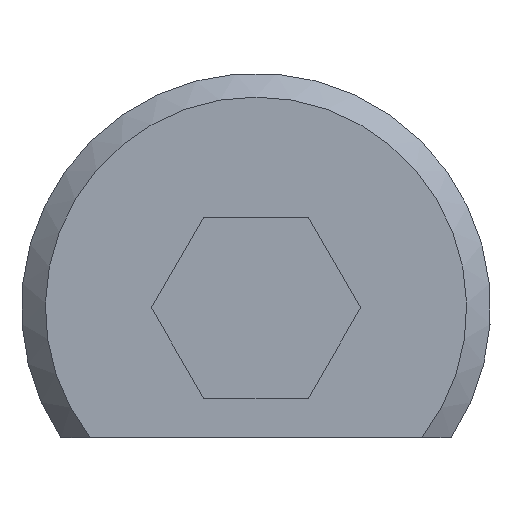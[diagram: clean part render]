
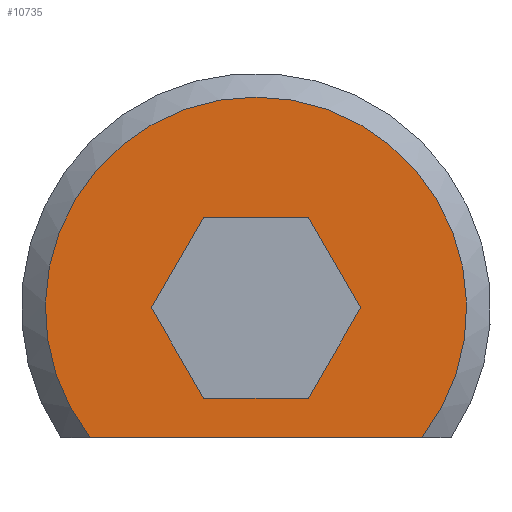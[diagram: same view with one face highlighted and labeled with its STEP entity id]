
A CAD part, left-side view. The second image highlights one B-rep face of the part: STEP entity #10735.
In plain terms, the highlighted planar face has unit normal (-1, 0, 0).
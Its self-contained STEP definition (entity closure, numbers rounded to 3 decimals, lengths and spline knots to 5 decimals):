
#2374 = CARTESIAN_POINT ( 'NONE',  ( -0.25, -0.26053, -0.20458 ) ) ;
#7805 = CARTESIAN_POINT ( 'NONE',  ( -0.25, -0.08223, 0.14242 ) ) ;
#7925 = CARTESIAN_POINT ( 'NONE',  ( -0.25, -0.16445, 0. ) ) ;
#10735 = ADVANCED_FACE ( 'NONE', ( #48228, #26675 ), #14291, .T. ) ;
#12114 = VERTEX_POINT ( 'NONE', #19685 ) ;
#14291 = PLANE ( 'NONE',  #78402 ) ;
#15123 = CARTESIAN_POINT ( 'NONE',  ( -0.25, 0.08223, 0.14242 ) ) ;
#15304 = DIRECTION ( 'NONE',  ( -1., 0., 0. ) ) ;
#15470 = VERTEX_POINT ( 'NONE', #93569 ) ;
#15492 = DIRECTION ( 'NONE',  ( 0., -1., 0. ) ) ;
#16878 = DIRECTION ( 'NONE',  ( 0., 0.5, -0.866 ) ) ;
#19685 = CARTESIAN_POINT ( 'NONE',  ( -0.25, -0.16445, 0. ) ) ;
#19991 = EDGE_CURVE ( 'NONE', #75004, #82267, #100222, .T. ) ;
#22116 = DIRECTION ( 'NONE',  ( 0., 0., 1. ) ) ;
#23734 = LINE ( 'NONE', #38439, #74412 ) ;
#24244 = ORIENTED_EDGE ( 'NONE', *, *, #19991, .F. ) ;
#25272 = CARTESIAN_POINT ( 'NONE',  ( -0.25, -0.08223, -0.14242 ) ) ;
#26675 = FACE_BOUND ( 'NONE', #87872, .T. ) ;
#28014 = EDGE_CURVE ( 'NONE', #12114, #42615, #59497, .T. ) ;
#29639 = ORIENTED_EDGE ( 'NONE', *, *, #64154, .T. ) ;
#32819 = EDGE_CURVE ( 'NONE', #15470, #101002, #70896, .T. ) ;
#33434 = EDGE_CURVE ( 'NONE', #91427, #12114, #78535, .T. ) ;
#33846 = DIRECTION ( 'NONE',  ( -1., 0., 0. ) ) ;
#35648 = CARTESIAN_POINT ( 'NONE',  ( -0.25, 0.16445, 0. ) ) ;
#36956 = ORIENTED_EDGE ( 'NONE', *, *, #32819, .T. ) ;
#37487 = CARTESIAN_POINT ( 'NONE',  ( -0.25, -0.08223, -0.14242 ) ) ;
#37988 = ORIENTED_EDGE ( 'NONE', *, *, #49142, .F. ) ;
#38439 = CARTESIAN_POINT ( 'NONE',  ( -0.25, 0.16445, 0. ) ) ;
#41132 = LINE ( 'NONE', #7805, #84249 ) ;
#42615 = VERTEX_POINT ( 'NONE', #70901 ) ;
#44824 = DIRECTION ( 'NONE',  ( 0., -0.5, 0.866 ) ) ;
#46846 = VECTOR ( 'NONE', #15492, 39.37008 ) ;
#48221 = DIRECTION ( 'NONE',  ( 0., 1., 0. ) ) ;
#48228 = FACE_OUTER_BOUND ( 'NONE', #63639, .T. ) ;
#49142 = EDGE_CURVE ( 'NONE', #82267, #62425, #23734, .T. ) ;
#51678 = CARTESIAN_POINT ( 'NONE',  ( -0.25, 0.08223, -0.14242 ) ) ;
#55062 = DIRECTION ( 'NONE',  ( 0., -0.5, -0.866 ) ) ;
#56161 = LINE ( 'NONE', #51678, #72602 ) ;
#56355 = AXIS2_PLACEMENT_3D ( 'NONE', #82709, #33846, #59314 ) ;
#56959 = VECTOR ( 'NONE', #44824, 39.37008 ) ;
#57149 = DIRECTION ( 'NONE',  ( 0., 0.5, 0.866 ) ) ;
#57428 = ORIENTED_EDGE ( 'NONE', *, *, #28014, .F. ) ;
#59314 = DIRECTION ( 'NONE',  ( 0., 0., 1. ) ) ;
#59497 = LINE ( 'NONE', #7925, #79833 ) ;
#62425 = VERTEX_POINT ( 'NONE', #81669 ) ;
#63639 = EDGE_LOOP ( 'NONE', ( #36956, #29639 ) ) ;
#64154 = EDGE_CURVE ( 'NONE', #101002, #15470, #103406, .T. ) ;
#69310 = DIRECTION ( 'NONE',  ( 0., -1., 0. ) ) ;
#69752 = VECTOR ( 'NONE', #16878, 39.37008 ) ;
#70896 = LINE ( 'NONE', #79967, #46846 ) ;
#70901 = CARTESIAN_POINT ( 'NONE',  ( -0.25, -0.08223, 0.14242 ) ) ;
#72602 = VECTOR ( 'NONE', #69310, 39.37008 ) ;
#73406 = CARTESIAN_POINT ( 'NONE',  ( -0.25, 0.08223, 0.14242 ) ) ;
#74412 = VECTOR ( 'NONE', #55062, 39.37008 ) ;
#75004 = VERTEX_POINT ( 'NONE', #73406 ) ;
#76286 = EDGE_CURVE ( 'NONE', #42615, #75004, #41132, .T. ) ;
#78402 = AXIS2_PLACEMENT_3D ( 'NONE', #87961, #15304, #22116 ) ;
#78535 = LINE ( 'NONE', #25272, #56959 ) ;
#79207 = ORIENTED_EDGE ( 'NONE', *, *, #76286, .F. ) ;
#79833 = VECTOR ( 'NONE', #57149, 39.37008 ) ;
#79967 = CARTESIAN_POINT ( 'NONE',  ( -0.25, 0.3068, -0.20458 ) ) ;
#81669 = CARTESIAN_POINT ( 'NONE',  ( -0.25, 0.08223, -0.14242 ) ) ;
#82267 = VERTEX_POINT ( 'NONE', #35648 ) ;
#82709 = CARTESIAN_POINT ( 'NONE',  ( -0.25, 0., 0. ) ) ;
#82754 = ORIENTED_EDGE ( 'NONE', *, *, #33434, .F. ) ;
#84249 = VECTOR ( 'NONE', #48221, 39.37008 ) ;
#87872 = EDGE_LOOP ( 'NONE', ( #91244, #37988, #24244, #79207, #57428, #82754 ) ) ;
#87961 = CARTESIAN_POINT ( 'NONE',  ( -0.25, 0., 0. ) ) ;
#91201 = EDGE_CURVE ( 'NONE', #62425, #91427, #56161, .T. ) ;
#91244 = ORIENTED_EDGE ( 'NONE', *, *, #91201, .F. ) ;
#91427 = VERTEX_POINT ( 'NONE', #37487 ) ;
#93569 = CARTESIAN_POINT ( 'NONE',  ( -0.25, 0.26053, -0.20458 ) ) ;
#100222 = LINE ( 'NONE', #15123, #69752 ) ;
#101002 = VERTEX_POINT ( 'NONE', #2374 ) ;
#103406 = CIRCLE ( 'NONE', #56355, 0.33125 ) ;
